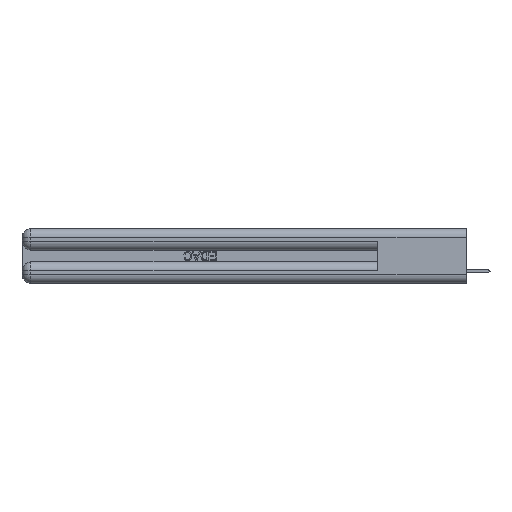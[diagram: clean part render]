
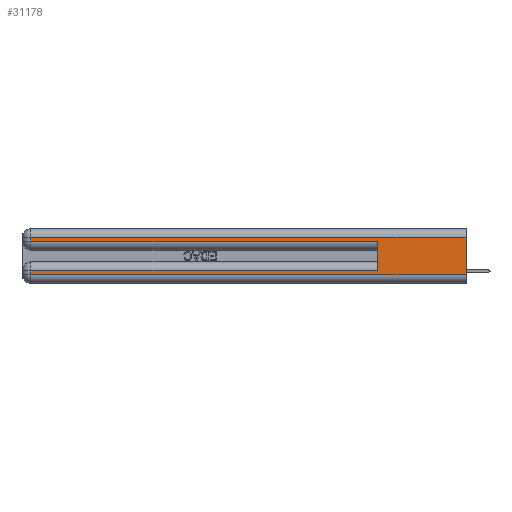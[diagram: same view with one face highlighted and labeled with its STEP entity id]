
A CAD part, left-side view. The second image highlights one B-rep face of the part: STEP entity #31178.
In plain terms, the highlighted planar face has unit normal (-1, 0, 0).
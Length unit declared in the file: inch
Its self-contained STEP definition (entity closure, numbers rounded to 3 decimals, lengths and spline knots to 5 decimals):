
#397 = AXIS2_PLACEMENT_3D ( 'NONE', #36153, #33308, #8293 ) ;
#1482 = ORIENTED_EDGE ( 'NONE', *, *, #33657, .T. ) ;
#1486 = CARTESIAN_POINT ( 'NONE',  ( 0., 2.94, 0.37 ) ) ;
#1927 = CARTESIAN_POINT ( 'NONE',  ( 0., 2.94, 0.285 ) ) ;
#2090 = ORIENTED_EDGE ( 'NONE', *, *, #5566, .T. ) ;
#2379 = DIRECTION ( 'NONE',  ( 0., -1., 0. ) ) ;
#2621 = LINE ( 'NONE', #35291, #14097 ) ;
#3756 = LINE ( 'NONE', #13980, #8605 ) ;
#3897 = ORIENTED_EDGE ( 'NONE', *, *, #19947, .T. ) ;
#5566 = EDGE_CURVE ( 'NONE', #21791, #31466, #26595, .T. ) ;
#6863 = ORIENTED_EDGE ( 'NONE', *, *, #31604, .T. ) ;
#7145 = VECTOR ( 'NONE', #22267, 39.37008 ) ;
#7195 = ORIENTED_EDGE ( 'NONE', *, *, #20737, .T. ) ;
#7290 = ORIENTED_EDGE ( 'NONE', *, *, #37356, .T. ) ;
#7606 = DIRECTION ( 'NONE',  ( 0., 0., -1. ) ) ;
#8293 = DIRECTION ( 'NONE',  ( 0., 0., -1. ) ) ;
#8599 = ORIENTED_EDGE ( 'NONE', *, *, #38404, .F. ) ;
#8605 = VECTOR ( 'NONE', #13842, 39.37008 ) ;
#9973 = CARTESIAN_POINT ( 'NONE',  ( 0., 0.6, 0.285 ) ) ;
#10101 = DIRECTION ( 'NONE',  ( 0., 0., -1. ) ) ;
#12299 = VECTOR ( 'NONE', #13540, 39.37008 ) ;
#13463 = FACE_OUTER_BOUND ( 'NONE', #24693, .T. ) ;
#13540 = DIRECTION ( 'NONE',  ( 0., 0., -1. ) ) ;
#13842 = DIRECTION ( 'NONE',  ( 0., 0., 1. ) ) ;
#13980 = CARTESIAN_POINT ( 'NONE',  ( 0., 0.6, 0.145 ) ) ;
#14097 = VECTOR ( 'NONE', #10101, 39.37008 ) ;
#14731 = CARTESIAN_POINT ( 'NONE',  ( 0., 2.94, 0.37 ) ) ;
#15066 = VERTEX_POINT ( 'NONE', #1927 ) ;
#15808 = DIRECTION ( 'NONE',  ( 0., 1., 0. ) ) ;
#16972 = EDGE_CURVE ( 'NONE', #22586, #20715, #3756, .T. ) ;
#18240 = LINE ( 'NONE', #31886, #20669 ) ;
#19305 = CARTESIAN_POINT ( 'NONE',  ( 0., 2.94, 0.31 ) ) ;
#19947 = EDGE_CURVE ( 'NONE', #25829, #24215, #38628, .T. ) ;
#20315 = CARTESIAN_POINT ( 'NONE',  ( 0., 0., 0.06 ) ) ;
#20669 = VECTOR ( 'NONE', #38195, 39.37008 ) ;
#20715 = VERTEX_POINT ( 'NONE', #9973 ) ;
#20737 = EDGE_CURVE ( 'NONE', #15066, #20715, #31820, .T. ) ;
#21791 = VERTEX_POINT ( 'NONE', #39280 ) ;
#22267 = DIRECTION ( 'NONE',  ( 0., -1., 0. ) ) ;
#22586 = VERTEX_POINT ( 'NONE', #35219 ) ;
#23749 = CARTESIAN_POINT ( 'NONE',  ( 0., 2.94, 0.085 ) ) ;
#24215 = VERTEX_POINT ( 'NONE', #32471 ) ;
#24693 = EDGE_LOOP ( 'NONE', ( #8599, #2090, #7290, #7195, #25234, #6863, #3897, #1482 ) ) ;
#25234 = ORIENTED_EDGE ( 'NONE', *, *, #16972, .F. ) ;
#25829 = VERTEX_POINT ( 'NONE', #23749 ) ;
#26105 = VECTOR ( 'NONE', #15808, 39.37008 ) ;
#26595 = LINE ( 'NONE', #34344, #26105 ) ;
#26817 = PLANE ( 'NONE',  #397 ) ;
#28607 = LINE ( 'NONE', #20315, #31517 ) ;
#30269 = VERTEX_POINT ( 'NONE', #37731 ) ;
#30478 = VECTOR ( 'NONE', #7606, 39.37008 ) ;
#31178 = ADVANCED_FACE ( 'NONE', ( #13463 ), #26817, .F. ) ;
#31466 = VERTEX_POINT ( 'NONE', #19305 ) ;
#31517 = VECTOR ( 'NONE', #2379, 39.37008 ) ;
#31604 = EDGE_CURVE ( 'NONE', #22586, #25829, #18240, .T. ) ;
#31820 = LINE ( 'NONE', #37530, #7145 ) ;
#31886 = CARTESIAN_POINT ( 'NONE',  ( 0., 0., 0.085 ) ) ;
#32471 = CARTESIAN_POINT ( 'NONE',  ( 0., 2.94, 0.06 ) ) ;
#33308 = DIRECTION ( 'NONE',  ( 1., 0., 0. ) ) ;
#33657 = EDGE_CURVE ( 'NONE', #24215, #30269, #28607, .T. ) ;
#34344 = CARTESIAN_POINT ( 'NONE',  ( 0., 0., 0.31 ) ) ;
#35219 = CARTESIAN_POINT ( 'NONE',  ( 0., 0.6, 0.085 ) ) ;
#35291 = CARTESIAN_POINT ( 'NONE',  ( 0., 0., 0.37 ) ) ;
#36153 = CARTESIAN_POINT ( 'NONE',  ( 0., 0., 0.37 ) ) ;
#36527 = LINE ( 'NONE', #1486, #12299 ) ;
#37356 = EDGE_CURVE ( 'NONE', #31466, #15066, #36527, .T. ) ;
#37530 = CARTESIAN_POINT ( 'NONE',  ( 0., 0., 0.285 ) ) ;
#37731 = CARTESIAN_POINT ( 'NONE',  ( 0., 0., 0.06 ) ) ;
#38195 = DIRECTION ( 'NONE',  ( 0., 1., 0. ) ) ;
#38404 = EDGE_CURVE ( 'NONE', #21791, #30269, #2621, .T. ) ;
#38628 = LINE ( 'NONE', #14731, #30478 ) ;
#39280 = CARTESIAN_POINT ( 'NONE',  ( 0., 0., 0.31 ) ) ;
